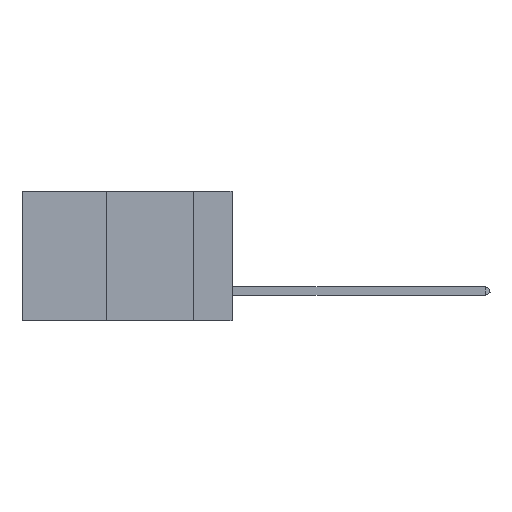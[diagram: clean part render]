
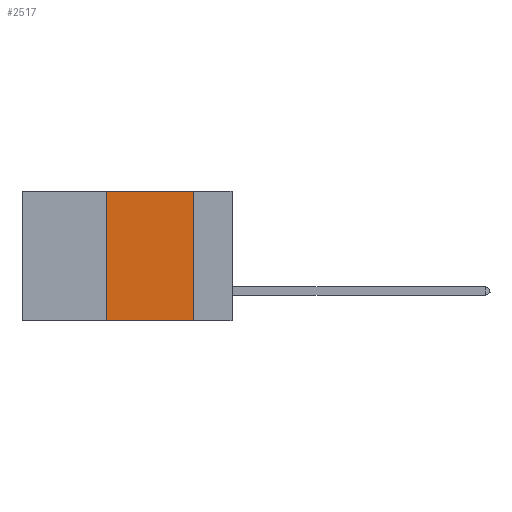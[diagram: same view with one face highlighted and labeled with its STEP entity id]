
A CAD part, left-side view. The second image highlights one B-rep face of the part: STEP entity #2517.
In plain terms, the highlighted planar face has unit normal (-1, 0, 0).
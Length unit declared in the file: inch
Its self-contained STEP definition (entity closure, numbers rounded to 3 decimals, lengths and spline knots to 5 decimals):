
#845 = DIRECTION ( 'NONE',  ( 0., 0., -1. ) ) ;
#1827 = VECTOR ( 'NONE', #39496, 39.37008 ) ;
#2517 = ADVANCED_FACE ( 'NONE', ( #32402 ), #24672, .F. ) ;
#4091 = VECTOR ( 'NONE', #34210, 39.37008 ) ;
#5288 = LINE ( 'NONE', #29281, #27666 ) ;
#9349 = EDGE_CURVE ( 'NONE', #15039, #21002, #35254, .T. ) ;
#10260 = EDGE_CURVE ( 'NONE', #24870, #21002, #5288, .T. ) ;
#15039 = VERTEX_POINT ( 'NONE', #30326 ) ;
#15476 = CARTESIAN_POINT ( 'NONE',  ( 0., 0.6, 0. ) ) ;
#15478 = EDGE_CURVE ( 'NONE', #29015, #15039, #19924, .T. ) ;
#16662 = EDGE_LOOP ( 'NONE', ( #22854, #43225, #26683, #20851 ) ) ;
#18680 = EDGE_CURVE ( 'NONE', #24870, #29015, #22261, .T. ) ;
#19924 = LINE ( 'NONE', #15476, #1827 ) ;
#20761 = AXIS2_PLACEMENT_3D ( 'NONE', #38240, #21262, #845 ) ;
#20851 = ORIENTED_EDGE ( 'NONE', *, *, #10260, .T. ) ;
#20878 = VECTOR ( 'NONE', #30682, 39.37008 ) ;
#21002 = VERTEX_POINT ( 'NONE', #43524 ) ;
#21262 = DIRECTION ( 'NONE',  ( 1., 0., 0. ) ) ;
#22261 = LINE ( 'NONE', #30631, #4091 ) ;
#22854 = ORIENTED_EDGE ( 'NONE', *, *, #9349, .F. ) ;
#24672 = PLANE ( 'NONE',  #20761 ) ;
#24870 = VERTEX_POINT ( 'NONE', #29145 ) ;
#26683 = ORIENTED_EDGE ( 'NONE', *, *, #18680, .F. ) ;
#27096 = CARTESIAN_POINT ( 'NONE',  ( 0., 0.11, 0. ) ) ;
#27666 = VECTOR ( 'NONE', #43008, 39.37008 ) ;
#29015 = VERTEX_POINT ( 'NONE', #43482 ) ;
#29145 = CARTESIAN_POINT ( 'NONE',  ( 0., 0.36, -0.37 ) ) ;
#29281 = CARTESIAN_POINT ( 'NONE',  ( 0., 0.6, -0.37 ) ) ;
#30326 = CARTESIAN_POINT ( 'NONE',  ( 0., 0.11, 0. ) ) ;
#30631 = CARTESIAN_POINT ( 'NONE',  ( 0., 0.36, 0. ) ) ;
#30682 = DIRECTION ( 'NONE',  ( 0., 0., -1. ) ) ;
#32402 = FACE_OUTER_BOUND ( 'NONE', #16662, .T. ) ;
#34210 = DIRECTION ( 'NONE',  ( 0., 0., 1. ) ) ;
#35254 = LINE ( 'NONE', #27096, #20878 ) ;
#38240 = CARTESIAN_POINT ( 'NONE',  ( 0., 0.6, 0. ) ) ;
#39496 = DIRECTION ( 'NONE',  ( 0., -1., 0. ) ) ;
#43008 = DIRECTION ( 'NONE',  ( 0., -1., 0. ) ) ;
#43225 = ORIENTED_EDGE ( 'NONE', *, *, #15478, .F. ) ;
#43482 = CARTESIAN_POINT ( 'NONE',  ( 0., 0.36, 0. ) ) ;
#43524 = CARTESIAN_POINT ( 'NONE',  ( 0., 0.11, -0.37 ) ) ;
